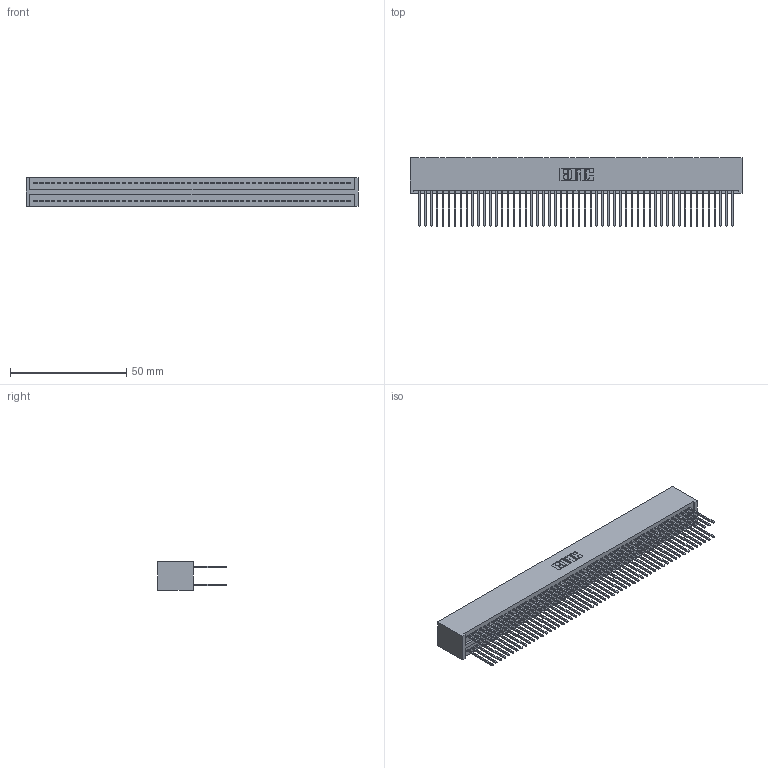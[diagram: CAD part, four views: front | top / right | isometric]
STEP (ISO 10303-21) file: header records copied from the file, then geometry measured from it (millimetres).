
FILE_DESCRIPTION (( 'STEP AP203' ), '1' );
FILE_NAME ('325-108-540-201.STEP', '2020-02-25T07:29:58', ( '' ), ( '' ), 'SwSTEP 2.0', 'SolidWorks 2016', '' );
FILE_SCHEMA (( 'CONFIG_CONTROL_DESIGN' ));
Length unit declared in the file: inch
Products named in the file (3): 325-108-540-201; 325-292-001_325-293-140; 325 Part_Lugless
Assembly tree (109 placements, depth 2):
  325-108-540-201
    325 Part_Lugless
    325-292-001_325-293-140  x108
Bounding box: 142.8 x 29.46 x 12.45 mm (x, y, z)
Volume: 19558.2 mm3; surface area: 26567.1 mm2
Topology: 109 solids, 109 shells, 5722 faces, 17027 edges, 11206 vertices
Faces by surface type: plane 3954, cylinder 1768
Entity records: 32929 total; most frequent: CARTESIAN_POINT 5442, ORIENTED_EDGE 5378, DIRECTION 4621, EDGE_CURVE 2689, VECTOR 2569, LINE 2569, VERTEX_POINT 1790, AXIS2_PLACEMENT_3D 1026
